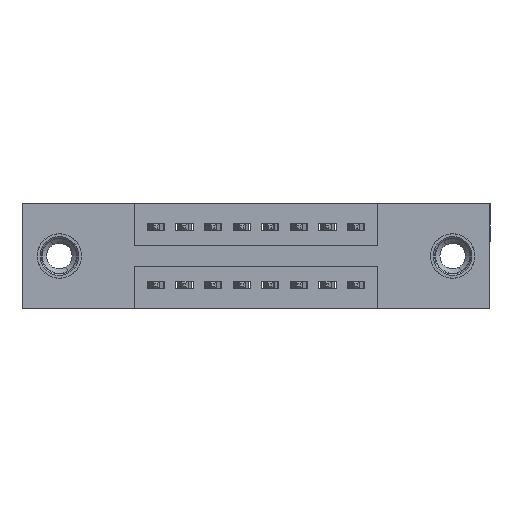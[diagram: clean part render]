
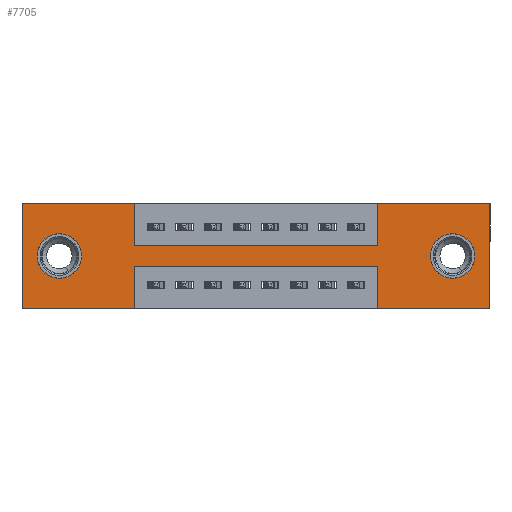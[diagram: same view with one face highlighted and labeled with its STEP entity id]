
A CAD part, front view. The second image highlights one B-rep face of the part: STEP entity #7705.
In plain terms, the highlighted planar face has unit normal (0, -1, 0).
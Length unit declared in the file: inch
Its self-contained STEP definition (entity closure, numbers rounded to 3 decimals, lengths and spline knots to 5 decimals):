
#57 = VERTEX_POINT ( 'NONE', #11137 ) ;
#169 = EDGE_CURVE ( 'NONE', #9788, #57, #10030, .T. ) ;
#170 = LINE ( 'NONE', #11773, #6347 ) ;
#264 = CARTESIAN_POINT ( 'NONE',  ( 1.505, 0., -0.185 ) ) ;
#391 = FACE_BOUND ( 'NONE', #4981, .T. ) ;
#516 = VECTOR ( 'NONE', #584, 39.37008 ) ;
#584 = DIRECTION ( 'NONE',  ( 0., 0., 1. ) ) ;
#757 = DIRECTION ( 'NONE',  ( 0., 0., -1. ) ) ;
#933 = VECTOR ( 'NONE', #10157, 39.37008 ) ;
#1023 = CARTESIAN_POINT ( 'NONE',  ( 1.2425, 0., 0. ) ) ;
#1041 = EDGE_CURVE ( 'NONE', #6530, #14830, #15330, .T. ) ;
#1158 = DIRECTION ( 'NONE',  ( 0., 1., 0. ) ) ;
#1413 = PLANE ( 'NONE',  #11222 ) ;
#1455 = CARTESIAN_POINT ( 'NONE',  ( 0.13, 0., -0.107 ) ) ;
#1473 = CARTESIAN_POINT ( 'NONE',  ( 1.635, 0., 0. ) ) ;
#1480 = DIRECTION ( 'NONE',  ( -1., 0., 0. ) ) ;
#1519 = DIRECTION ( 'NONE',  ( 0., 0., -1. ) ) ;
#1641 = DIRECTION ( 'NONE',  ( 0., 0., -1. ) ) ;
#1755 = EDGE_CURVE ( 'NONE', #1979, #4529, #170, .T. ) ;
#1806 = CARTESIAN_POINT ( 'NONE',  ( 0.13, 0., -0.263 ) ) ;
#1979 = VERTEX_POINT ( 'NONE', #5159 ) ;
#2084 = EDGE_LOOP ( 'NONE', ( #9488, #3741, #7351, #6091, #3051, #14097, #8107, #7592, #14139, #3918, #15036, #13279 ) ) ;
#2234 = VERTEX_POINT ( 'NONE', #1806 ) ;
#2498 = EDGE_CURVE ( 'NONE', #6259, #1979, #15281, .T. ) ;
#2604 = AXIS2_PLACEMENT_3D ( 'NONE', #14256, #7131, #15428 ) ;
#2708 = EDGE_CURVE ( 'NONE', #10971, #13493, #3474, .T. ) ;
#2925 = EDGE_CURVE ( 'NONE', #13493, #13637, #10528, .T. ) ;
#2986 = DIRECTION ( 'NONE',  ( 0., 0., -1. ) ) ;
#3010 = EDGE_LOOP ( 'NONE', ( #14966, #7454 ) ) ;
#3051 = ORIENTED_EDGE ( 'NONE', *, *, #2925, .F. ) ;
#3168 = EDGE_CURVE ( 'NONE', #13637, #6259, #7324, .T. ) ;
#3474 = LINE ( 'NONE', #15323, #933 ) ;
#3741 = ORIENTED_EDGE ( 'NONE', *, *, #1755, .F. ) ;
#3918 = ORIENTED_EDGE ( 'NONE', *, *, #169, .F. ) ;
#4047 = VECTOR ( 'NONE', #10915, 39.37008 ) ;
#4313 = VECTOR ( 'NONE', #8912, 39.37008 ) ;
#4441 = LINE ( 'NONE', #10220, #4824 ) ;
#4529 = VERTEX_POINT ( 'NONE', #9150 ) ;
#4824 = VECTOR ( 'NONE', #1641, 39.37008 ) ;
#4907 = DIRECTION ( 'NONE',  ( 0., 1., 0. ) ) ;
#4974 = LINE ( 'NONE', #8168, #14532 ) ;
#4981 = EDGE_LOOP ( 'NONE', ( #11631, #9976 ) ) ;
#5037 = VECTOR ( 'NONE', #1480, 39.37008 ) ;
#5159 = CARTESIAN_POINT ( 'NONE',  ( 1.2425, 0., -0.22 ) ) ;
#5215 = CARTESIAN_POINT ( 'NONE',  ( 1.2425, 0., -0.37 ) ) ;
#5217 = CIRCLE ( 'NONE', #12501, 0.078 ) ;
#5306 = DIRECTION ( 'NONE',  ( 0., 0., 1. ) ) ;
#6091 = ORIENTED_EDGE ( 'NONE', *, *, #3168, .F. ) ;
#6259 = VERTEX_POINT ( 'NONE', #9717 ) ;
#6347 = VECTOR ( 'NONE', #12402, 39.37008 ) ;
#6530 = VERTEX_POINT ( 'NONE', #6600 ) ;
#6600 = CARTESIAN_POINT ( 'NONE',  ( 0.3925, 0., -0.15 ) ) ;
#6731 = VERTEX_POINT ( 'NONE', #11801 ) ;
#6907 = VECTOR ( 'NONE', #2986, 39.37008 ) ;
#6932 = VECTOR ( 'NONE', #12557, 39.37008 ) ;
#6964 = FACE_BOUND ( 'NONE', #3010, .T. ) ;
#7131 = DIRECTION ( 'NONE',  ( 0., 1., 0. ) ) ;
#7241 = AXIS2_PLACEMENT_3D ( 'NONE', #8546, #1158, #9724 ) ;
#7244 = CARTESIAN_POINT ( 'NONE',  ( 1.505, 0., -0.107 ) ) ;
#7324 = LINE ( 'NONE', #9701, #4047 ) ;
#7351 = ORIENTED_EDGE ( 'NONE', *, *, #2498, .F. ) ;
#7454 = ORIENTED_EDGE ( 'NONE', *, *, #10343, .T. ) ;
#7592 = ORIENTED_EDGE ( 'NONE', *, *, #1041, .F. ) ;
#7616 = DIRECTION ( 'NONE',  ( 0., 0., -1. ) ) ;
#7705 = ADVANCED_FACE ( 'NONE', ( #6964, #391, #13328 ), #1413, .T. ) ;
#7791 = CARTESIAN_POINT ( 'NONE',  ( 1.635, 0., -0.37 ) ) ;
#7869 = CARTESIAN_POINT ( 'NONE',  ( 1.635, 0., 0. ) ) ;
#8107 = ORIENTED_EDGE ( 'NONE', *, *, #13622, .F. ) ;
#8144 = EDGE_CURVE ( 'NONE', #8588, #6731, #5217, .T. ) ;
#8168 = CARTESIAN_POINT ( 'NONE',  ( 0.3925, 0., -0.37 ) ) ;
#8329 = LINE ( 'NONE', #10066, #5037 ) ;
#8546 = CARTESIAN_POINT ( 'NONE',  ( 0.13, 0., -0.185 ) ) ;
#8588 = VERTEX_POINT ( 'NONE', #7244 ) ;
#8904 = DIRECTION ( 'NONE',  ( 0., 1., 0. ) ) ;
#8912 = DIRECTION ( 'NONE',  ( 1., 0., 0. ) ) ;
#9038 = VECTOR ( 'NONE', #5306, 39.37008 ) ;
#9080 = VECTOR ( 'NONE', #11743, 39.37008 ) ;
#9150 = CARTESIAN_POINT ( 'NONE',  ( 0.3925, 0., -0.22 ) ) ;
#9177 = CARTESIAN_POINT ( 'NONE',  ( 0., 0., 0. ) ) ;
#9264 = CIRCLE ( 'NONE', #7241, 0.078 ) ;
#9488 = ORIENTED_EDGE ( 'NONE', *, *, #14298, .F. ) ;
#9701 = CARTESIAN_POINT ( 'NONE',  ( 0., 0., -0.37 ) ) ;
#9717 = CARTESIAN_POINT ( 'NONE',  ( 1.2425, 0., -0.37 ) ) ;
#9724 = DIRECTION ( 'NONE',  ( 0., 0., 1. ) ) ;
#9788 = VERTEX_POINT ( 'NONE', #12139 ) ;
#9976 = ORIENTED_EDGE ( 'NONE', *, *, #12141, .T. ) ;
#10030 = LINE ( 'NONE', #9177, #4313 ) ;
#10066 = CARTESIAN_POINT ( 'NONE',  ( 0., 0., -0.37 ) ) ;
#10157 = DIRECTION ( 'NONE',  ( 1., 0., 0. ) ) ;
#10220 = CARTESIAN_POINT ( 'NONE',  ( 0.3925, 0., 0. ) ) ;
#10343 = EDGE_CURVE ( 'NONE', #6731, #8588, #11623, .T. ) ;
#10378 = VERTEX_POINT ( 'NONE', #13386 ) ;
#10412 = CARTESIAN_POINT ( 'NONE',  ( 0., 0., 0. ) ) ;
#10528 = LINE ( 'NONE', #7869, #6907 ) ;
#10560 = CARTESIAN_POINT ( 'NONE',  ( 0.3925, 0., -0.15 ) ) ;
#10915 = DIRECTION ( 'NONE',  ( -1., 0., 0. ) ) ;
#10971 = VERTEX_POINT ( 'NONE', #1023 ) ;
#11137 = CARTESIAN_POINT ( 'NONE',  ( 0.3925, 0., 0. ) ) ;
#11222 = AXIS2_PLACEMENT_3D ( 'NONE', #12381, #14701, #7616 ) ;
#11623 = CIRCLE ( 'NONE', #15142, 0.078 ) ;
#11631 = ORIENTED_EDGE ( 'NONE', *, *, #14384, .T. ) ;
#11704 = EDGE_CURVE ( 'NONE', #15509, #10378, #8329, .T. ) ;
#11743 = DIRECTION ( 'NONE',  ( 1., 0., 0. ) ) ;
#11773 = CARTESIAN_POINT ( 'NONE',  ( 0.3925, 0., -0.22 ) ) ;
#11801 = CARTESIAN_POINT ( 'NONE',  ( 1.505, 0., -0.263 ) ) ;
#12139 = CARTESIAN_POINT ( 'NONE',  ( 0., 0., 0. ) ) ;
#12141 = EDGE_CURVE ( 'NONE', #2234, #12299, #9264, .T. ) ;
#12166 = CARTESIAN_POINT ( 'NONE',  ( 1.505, 0., -0.185 ) ) ;
#12299 = VERTEX_POINT ( 'NONE', #1455 ) ;
#12381 = CARTESIAN_POINT ( 'NONE',  ( 0., 0., -0.37 ) ) ;
#12402 = DIRECTION ( 'NONE',  ( -1., 0., 0. ) ) ;
#12501 = AXIS2_PLACEMENT_3D ( 'NONE', #264, #8904, #1519 ) ;
#12557 = DIRECTION ( 'NONE',  ( 0., 0., 1. ) ) ;
#12726 = CIRCLE ( 'NONE', #2604, 0.078 ) ;
#13279 = ORIENTED_EDGE ( 'NONE', *, *, #11704, .F. ) ;
#13299 = LINE ( 'NONE', #14813, #6932 ) ;
#13328 = FACE_OUTER_BOUND ( 'NONE', #2084, .T. ) ;
#13336 = DIRECTION ( 'NONE',  ( 0., 0., -1. ) ) ;
#13386 = CARTESIAN_POINT ( 'NONE',  ( 0., 0., -0.37 ) ) ;
#13436 = LINE ( 'NONE', #10412, #516 ) ;
#13493 = VERTEX_POINT ( 'NONE', #1473 ) ;
#13567 = EDGE_CURVE ( 'NONE', #57, #6530, #4441, .T. ) ;
#13622 = EDGE_CURVE ( 'NONE', #14830, #10971, #13299, .T. ) ;
#13637 = VERTEX_POINT ( 'NONE', #7791 ) ;
#13942 = CARTESIAN_POINT ( 'NONE',  ( 1.2425, 0., -0.15 ) ) ;
#14097 = ORIENTED_EDGE ( 'NONE', *, *, #2708, .F. ) ;
#14139 = ORIENTED_EDGE ( 'NONE', *, *, #13567, .F. ) ;
#14256 = CARTESIAN_POINT ( 'NONE',  ( 0.13, 0., -0.185 ) ) ;
#14298 = EDGE_CURVE ( 'NONE', #4529, #15509, #4974, .T. ) ;
#14384 = EDGE_CURVE ( 'NONE', #12299, #2234, #12726, .T. ) ;
#14532 = VECTOR ( 'NONE', #757, 39.37008 ) ;
#14701 = DIRECTION ( 'NONE',  ( 0., -1., 0. ) ) ;
#14813 = CARTESIAN_POINT ( 'NONE',  ( 1.2425, 0., 0. ) ) ;
#14821 = EDGE_CURVE ( 'NONE', #10378, #9788, #13436, .T. ) ;
#14830 = VERTEX_POINT ( 'NONE', #13942 ) ;
#14966 = ORIENTED_EDGE ( 'NONE', *, *, #8144, .T. ) ;
#15036 = ORIENTED_EDGE ( 'NONE', *, *, #14821, .F. ) ;
#15131 = CARTESIAN_POINT ( 'NONE',  ( 0.3925, 0., -0.37 ) ) ;
#15142 = AXIS2_PLACEMENT_3D ( 'NONE', #12166, #4907, #13336 ) ;
#15281 = LINE ( 'NONE', #5215, #9038 ) ;
#15323 = CARTESIAN_POINT ( 'NONE',  ( 0., 0., 0. ) ) ;
#15330 = LINE ( 'NONE', #10560, #9080 ) ;
#15428 = DIRECTION ( 'NONE',  ( 0., 0., 1. ) ) ;
#15509 = VERTEX_POINT ( 'NONE', #15131 ) ;
